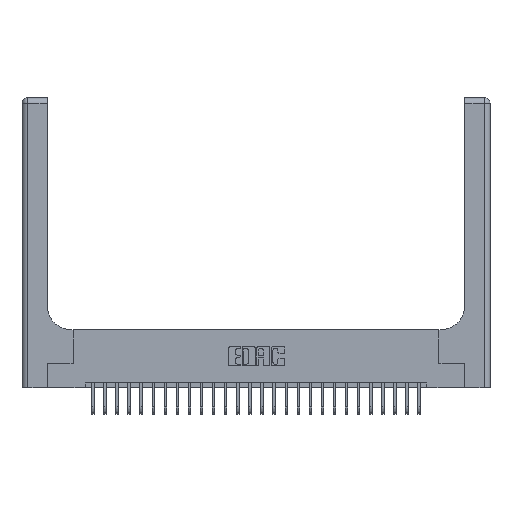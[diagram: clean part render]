
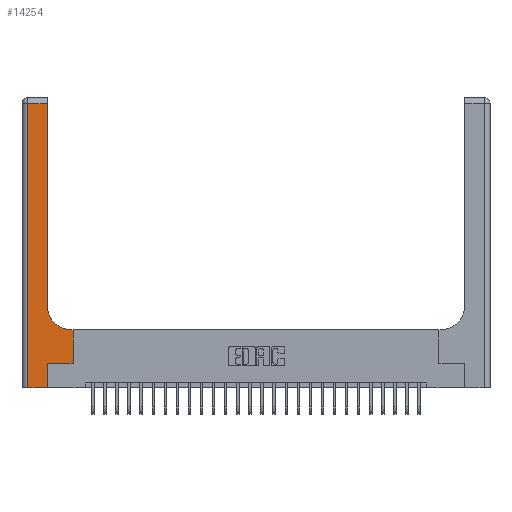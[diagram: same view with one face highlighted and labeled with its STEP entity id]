
A CAD part, top view. The second image highlights one B-rep face of the part: STEP entity #14254.
In plain terms, the highlighted planar face has unit normal (0, 0, 1).
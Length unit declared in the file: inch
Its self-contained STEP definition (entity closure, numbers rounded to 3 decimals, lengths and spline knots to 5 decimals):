
#435 = VECTOR ( 'NONE', #19805, 39.37008 ) ;
#943 = DIRECTION ( 'NONE',  ( -1., 0., 0. ) ) ;
#1065 = VERTEX_POINT ( 'NONE', #10698 ) ;
#1287 = VERTEX_POINT ( 'NONE', #8733 ) ;
#1864 = VECTOR ( 'NONE', #18687, 39.37008 ) ;
#1960 = LINE ( 'NONE', #12711, #7170 ) ;
#2118 = AXIS2_PLACEMENT_3D ( 'NONE', #11497, #20023, #943 ) ;
#2172 = DIRECTION ( 'NONE',  ( 0., 1., 0. ) ) ;
#2384 = VERTEX_POINT ( 'NONE', #22440 ) ;
#3184 = LINE ( 'NONE', #9420, #435 ) ;
#3772 = CARTESIAN_POINT ( 'NONE',  ( 0.06, 0., 0.37 ) ) ;
#4513 = LINE ( 'NONE', #23777, #23121 ) ;
#5087 = FACE_OUTER_BOUND ( 'NONE', #22793, .T. ) ;
#5241 = EDGE_CURVE ( 'NONE', #23673, #12397, #19973, .T. ) ;
#5872 = CARTESIAN_POINT ( 'NONE',  ( 0.26, 3., 0.37 ) ) ;
#6161 = VECTOR ( 'NONE', #10089, 39.37008 ) ;
#7163 = LINE ( 'NONE', #21969, #11312 ) ;
#7170 = VECTOR ( 'NONE', #21323, 39.37008 ) ;
#7429 = ORIENTED_EDGE ( 'NONE', *, *, #21250, .T. ) ;
#8120 = CIRCLE ( 'NONE', #27317, 0.25 ) ;
#8517 = ORIENTED_EDGE ( 'NONE', *, *, #5241, .T. ) ;
#8733 = CARTESIAN_POINT ( 'NONE',  ( 0.528, 0.25, 0.37 ) ) ;
#8791 = ORIENTED_EDGE ( 'NONE', *, *, #16491, .T. ) ;
#9420 = CARTESIAN_POINT ( 'NONE',  ( 0.265, 0.25, 0.37 ) ) ;
#9959 = CARTESIAN_POINT ( 'NONE',  ( 0.06, 2.94, 0.37 ) ) ;
#10089 = DIRECTION ( 'NONE',  ( -1., 0., 0. ) ) ;
#10128 = CARTESIAN_POINT ( 'NONE',  ( 0.06, 3., 0.37 ) ) ;
#10698 = CARTESIAN_POINT ( 'NONE',  ( 0.26, 0.85, 0.37 ) ) ;
#11096 = VECTOR ( 'NONE', #14566, 39.37008 ) ;
#11312 = VECTOR ( 'NONE', #21835, 39.37008 ) ;
#11497 = CARTESIAN_POINT ( 'NONE',  ( 0., 3., 0.37 ) ) ;
#11651 = LINE ( 'NONE', #26757, #6161 ) ;
#11660 = VERTEX_POINT ( 'NONE', #13731 ) ;
#12397 = VERTEX_POINT ( 'NONE', #13859 ) ;
#12414 = DIRECTION ( 'NONE',  ( 1., 0., 0. ) ) ;
#12566 = LINE ( 'NONE', #10128, #1864 ) ;
#12711 = CARTESIAN_POINT ( 'NONE',  ( 0.528, 0.25, 0.37 ) ) ;
#13639 = PLANE ( 'NONE',  #2118 ) ;
#13722 = CARTESIAN_POINT ( 'NONE',  ( 0.26, 0.6, 0.37 ) ) ;
#13731 = CARTESIAN_POINT ( 'NONE',  ( 0.26, 2.94, 0.37 ) ) ;
#13859 = CARTESIAN_POINT ( 'NONE',  ( 0.51, 0.6, 0.37 ) ) ;
#14230 = CARTESIAN_POINT ( 'NONE',  ( 0.51, 0.85, 0.37 ) ) ;
#14254 = ADVANCED_FACE ( 'NONE', ( #5087 ), #13639, .F. ) ;
#14566 = DIRECTION ( 'NONE',  ( 0., 1., 0. ) ) ;
#15293 = VECTOR ( 'NONE', #19705, 39.37008 ) ;
#16233 = EDGE_CURVE ( 'NONE', #26507, #2384, #4513, .T. ) ;
#16491 = EDGE_CURVE ( 'NONE', #11660, #23904, #11651, .T. ) ;
#16537 = LINE ( 'NONE', #5872, #11096 ) ;
#16673 = ORIENTED_EDGE ( 'NONE', *, *, #22266, .T. ) ;
#16842 = EDGE_CURVE ( 'NONE', #2384, #1287, #3184, .T. ) ;
#18687 = DIRECTION ( 'NONE',  ( 0., -1., 0. ) ) ;
#19022 = EDGE_CURVE ( 'NONE', #1065, #11660, #16537, .T. ) ;
#19308 = VERTEX_POINT ( 'NONE', #3772 ) ;
#19705 = DIRECTION ( 'NONE',  ( -1., 0., 0. ) ) ;
#19805 = DIRECTION ( 'NONE',  ( 1., 0., 0. ) ) ;
#19973 = LINE ( 'NONE', #13722, #15293 ) ;
#20023 = DIRECTION ( 'NONE',  ( 0., 0., -1. ) ) ;
#20146 = ORIENTED_EDGE ( 'NONE', *, *, #21286, .T. ) ;
#20168 = CARTESIAN_POINT ( 'NONE',  ( 0.265, 0., 0.37 ) ) ;
#21250 = EDGE_CURVE ( 'NONE', #23904, #19308, #12566, .T. ) ;
#21286 = EDGE_CURVE ( 'NONE', #1287, #23673, #1960, .T. ) ;
#21323 = DIRECTION ( 'NONE',  ( 0., 1., 0. ) ) ;
#21835 = DIRECTION ( 'NONE',  ( 1., 0., 0. ) ) ;
#21969 = CARTESIAN_POINT ( 'NONE',  ( 0., 0., 0.37 ) ) ;
#22266 = EDGE_CURVE ( 'NONE', #12397, #1065, #8120, .T. ) ;
#22440 = CARTESIAN_POINT ( 'NONE',  ( 0.265, 0.25, 0.37 ) ) ;
#22793 = EDGE_LOOP ( 'NONE', ( #27347, #8791, #7429, #24474, #25281, #26137, #20146, #8517, #16673 ) ) ;
#22999 = DIRECTION ( 'NONE',  ( 0., 0., -1. ) ) ;
#23121 = VECTOR ( 'NONE', #2172, 39.37008 ) ;
#23673 = VERTEX_POINT ( 'NONE', #25301 ) ;
#23777 = CARTESIAN_POINT ( 'NONE',  ( 0.265, 0., 0.37 ) ) ;
#23904 = VERTEX_POINT ( 'NONE', #9959 ) ;
#24474 = ORIENTED_EDGE ( 'NONE', *, *, #26482, .T. ) ;
#25281 = ORIENTED_EDGE ( 'NONE', *, *, #16233, .T. ) ;
#25301 = CARTESIAN_POINT ( 'NONE',  ( 0.528, 0.6, 0.37 ) ) ;
#26137 = ORIENTED_EDGE ( 'NONE', *, *, #16842, .T. ) ;
#26482 = EDGE_CURVE ( 'NONE', #19308, #26507, #7163, .T. ) ;
#26507 = VERTEX_POINT ( 'NONE', #20168 ) ;
#26757 = CARTESIAN_POINT ( 'NONE',  ( 0., 2.94, 0.37 ) ) ;
#27317 = AXIS2_PLACEMENT_3D ( 'NONE', #14230, #22999, #12414 ) ;
#27347 = ORIENTED_EDGE ( 'NONE', *, *, #19022, .T. ) ;
